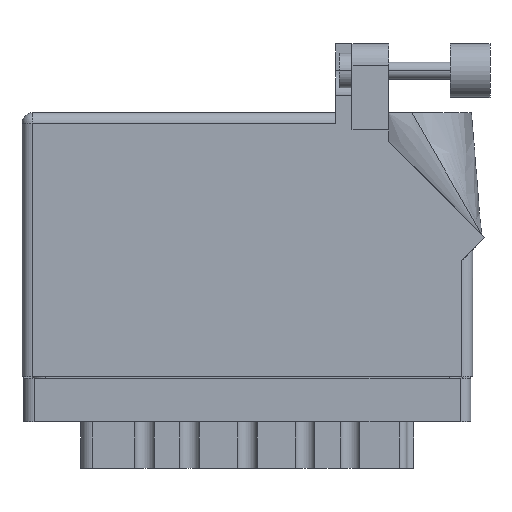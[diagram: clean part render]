
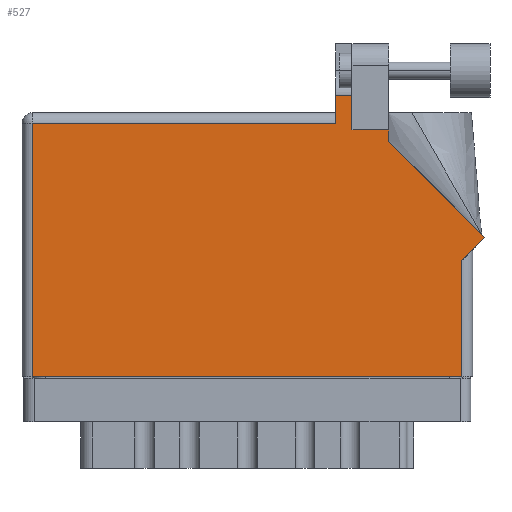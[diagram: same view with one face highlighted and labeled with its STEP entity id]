
A CAD part, front view. The second image highlights one B-rep face of the part: STEP entity #527.
In plain terms, the highlighted face is planar.
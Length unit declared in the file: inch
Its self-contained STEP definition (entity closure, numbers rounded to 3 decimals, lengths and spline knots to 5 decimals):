
#202 = LINE ( 'NONE', #49456, #15189 ) ;
#527 = ADVANCED_FACE ( 'NONE', ( #15389 ), #19867, .F. ) ;
#844 = EDGE_CURVE ( 'NONE', #41298, #24526, #45916, .T. ) ;
#1333 = CARTESIAN_POINT ( 'NONE',  ( 0.062, 0., 0. ) ) ;
#1377 = CARTESIAN_POINT ( 'NONE',  ( 1.913, 1.43, 0. ) ) ;
#2252 = ORIENTED_EDGE ( 'NONE', *, *, #9071, .T. ) ;
#2667 = LINE ( 'NONE', #34524, #28000 ) ;
#2992 = CARTESIAN_POINT ( 'NONE',  ( 1.819, 1.53, 0. ) ) ;
#3289 = CARTESIAN_POINT ( 'NONE',  ( 1.913, 1.43, 0. ) ) ;
#3355 = CARTESIAN_POINT ( 'NONE',  ( 2.68271, 0.80771, 0. ) ) ;
#3664 = DIRECTION ( 'NONE',  ( -1., 0., 0. ) ) ;
#3787 = VERTEX_POINT ( 'NONE', #13555 ) ;
#5615 = ORIENTED_EDGE ( 'NONE', *, *, #27315, .T. ) ;
#5771 = CARTESIAN_POINT ( 'NONE',  ( 2.55, 0., 0. ) ) ;
#6553 = CARTESIAN_POINT ( 'NONE',  ( 2.68271, 0.80771, 0. ) ) ;
#7386 = CARTESIAN_POINT ( 'NONE',  ( 1.913, 1.6315, 0. ) ) ;
#9071 = EDGE_CURVE ( 'NONE', #51226, #21111, #22725, .T. ) ;
#9334 = CARTESIAN_POINT ( 'NONE',  ( 1.819, 1.468, 0. ) ) ;
#9513 = CARTESIAN_POINT ( 'NONE',  ( 0., 0., 0. ) ) ;
#10589 = CARTESIAN_POINT ( 'NONE',  ( 2.612, 0.737, 0. ) ) ;
#10590 = ORIENTED_EDGE ( 'NONE', *, *, #33650, .T. ) ;
#11016 = VERTEX_POINT ( 'NONE', #51100 ) ;
#11277 = VECTOR ( 'NONE', #47327, 39.37008 ) ;
#11330 = DIRECTION ( 'NONE',  ( 0., 1., 0. ) ) ;
#13067 = VERTEX_POINT ( 'NONE', #5771 ) ;
#13555 = CARTESIAN_POINT ( 'NONE',  ( 2.55, 0.675, 0. ) ) ;
#13801 = EDGE_LOOP ( 'NONE', ( #5615, #33613, #10590, #48529, #2252, #41652, #22778, #53859, #33970, #31487, #44799 ) ) ;
#14125 = DIRECTION ( 'NONE',  ( -1., 0., 0. ) ) ;
#14722 = VECTOR ( 'NONE', #17300, 39.37008 ) ;
#15087 = EDGE_CURVE ( 'NONE', #13067, #3787, #202, .T. ) ;
#15189 = VECTOR ( 'NONE', #32194, 39.37008 ) ;
#15389 = FACE_OUTER_BOUND ( 'NONE', #13801, .T. ) ;
#15867 = EDGE_CURVE ( 'NONE', #23152, #11016, #24804, .T. ) ;
#16186 = EDGE_CURVE ( 'NONE', #19394, #51226, #2667, .T. ) ;
#16773 = CARTESIAN_POINT ( 'NONE',  ( 2.126, 1.36442, 0. ) ) ;
#17283 = EDGE_CURVE ( 'NONE', #24526, #37936, #53283, .T. ) ;
#17300 = DIRECTION ( 'NONE',  ( 0., 1., 0. ) ) ;
#17649 = VECTOR ( 'NONE', #44370, 39.37008 ) ;
#19069 = DIRECTION ( 'NONE',  ( 0.707, 0.707, 0. ) ) ;
#19394 = VERTEX_POINT ( 'NONE', #9334 ) ;
#19756 = CARTESIAN_POINT ( 'NONE',  ( 2.24377, 1.6315, 0. ) ) ;
#19867 = PLANE ( 'NONE',  #42864 ) ;
#20812 = VECTOR ( 'NONE', #46534, 39.37008 ) ;
#21111 = VERTEX_POINT ( 'NONE', #1333 ) ;
#22125 = LINE ( 'NONE', #3355, #52133 ) ;
#22725 = LINE ( 'NONE', #25914, #20812 ) ;
#22778 = ORIENTED_EDGE ( 'NONE', *, *, #15087, .T. ) ;
#23144 = DIRECTION ( 'NONE',  ( 0., -1., 0. ) ) ;
#23152 = VERTEX_POINT ( 'NONE', #7386 ) ;
#24018 = CARTESIAN_POINT ( 'NONE',  ( 2.126, 1.43, 0. ) ) ;
#24526 = VERTEX_POINT ( 'NONE', #50303 ) ;
#24804 = LINE ( 'NONE', #19756, #17649 ) ;
#25914 = CARTESIAN_POINT ( 'NONE',  ( 0.062, 0., 0. ) ) ;
#26080 = VERTEX_POINT ( 'NONE', #6553 ) ;
#27315 = EDGE_CURVE ( 'NONE', #37936, #23152, #45844, .T. ) ;
#27706 = CARTESIAN_POINT ( 'NONE',  ( 0., 1.53, 0. ) ) ;
#27871 = CARTESIAN_POINT ( 'NONE',  ( 2.126, 1.36442, 0. ) ) ;
#28000 = VECTOR ( 'NONE', #14125, 39.37008 ) ;
#28732 = VECTOR ( 'NONE', #23144, 39.37008 ) ;
#31487 = ORIENTED_EDGE ( 'NONE', *, *, #844, .T. ) ;
#32194 = DIRECTION ( 'NONE',  ( 0., 1., 0. ) ) ;
#32306 = EDGE_CURVE ( 'NONE', #3787, #26080, #38671, .T. ) ;
#33398 = LINE ( 'NONE', #9513, #11277 ) ;
#33613 = ORIENTED_EDGE ( 'NONE', *, *, #15867, .T. ) ;
#33650 = EDGE_CURVE ( 'NONE', #11016, #19394, #48963, .T. ) ;
#33970 = ORIENTED_EDGE ( 'NONE', *, *, #38290, .T. ) ;
#34524 = CARTESIAN_POINT ( 'NONE',  ( 0., 1.468, 0. ) ) ;
#36313 = DIRECTION ( 'NONE',  ( 0., 0., -1. ) ) ;
#36834 = DIRECTION ( 'NONE',  ( -0.707, 0.707, 0. ) ) ;
#37936 = VERTEX_POINT ( 'NONE', #1377 ) ;
#38290 = EDGE_CURVE ( 'NONE', #26080, #41298, #22125, .T. ) ;
#38671 = LINE ( 'NONE', #10589, #45192 ) ;
#40233 = VECTOR ( 'NONE', #3664, 39.37008 ) ;
#41298 = VERTEX_POINT ( 'NONE', #27871 ) ;
#41652 = ORIENTED_EDGE ( 'NONE', *, *, #49936, .T. ) ;
#42864 = AXIS2_PLACEMENT_3D ( 'NONE', #27706, #36313, #52868 ) ;
#44370 = DIRECTION ( 'NONE',  ( -1., 0., 0. ) ) ;
#44799 = ORIENTED_EDGE ( 'NONE', *, *, #17283, .T. ) ;
#45192 = VECTOR ( 'NONE', #19069, 39.37008 ) ;
#45844 = LINE ( 'NONE', #3289, #50390 ) ;
#45916 = LINE ( 'NONE', #16773, #14722 ) ;
#46534 = DIRECTION ( 'NONE',  ( 0., -1., 0. ) ) ;
#47327 = DIRECTION ( 'NONE',  ( 1., 0., 0. ) ) ;
#48529 = ORIENTED_EDGE ( 'NONE', *, *, #16186, .T. ) ;
#48749 = CARTESIAN_POINT ( 'NONE',  ( 0.062, 1.468, 0. ) ) ;
#48963 = LINE ( 'NONE', #2992, #28732 ) ;
#49456 = CARTESIAN_POINT ( 'NONE',  ( 2.55, 0.737, 0. ) ) ;
#49936 = EDGE_CURVE ( 'NONE', #21111, #13067, #33398, .T. ) ;
#50303 = CARTESIAN_POINT ( 'NONE',  ( 2.126, 1.43, 0. ) ) ;
#50390 = VECTOR ( 'NONE', #11330, 39.37008 ) ;
#51100 = CARTESIAN_POINT ( 'NONE',  ( 1.819, 1.6315, 0. ) ) ;
#51226 = VERTEX_POINT ( 'NONE', #48749 ) ;
#52133 = VECTOR ( 'NONE', #36834, 39.37008 ) ;
#52868 = DIRECTION ( 'NONE',  ( -1., 0., 0. ) ) ;
#53283 = LINE ( 'NONE', #24018, #40233 ) ;
#53859 = ORIENTED_EDGE ( 'NONE', *, *, #32306, .T. ) ;
